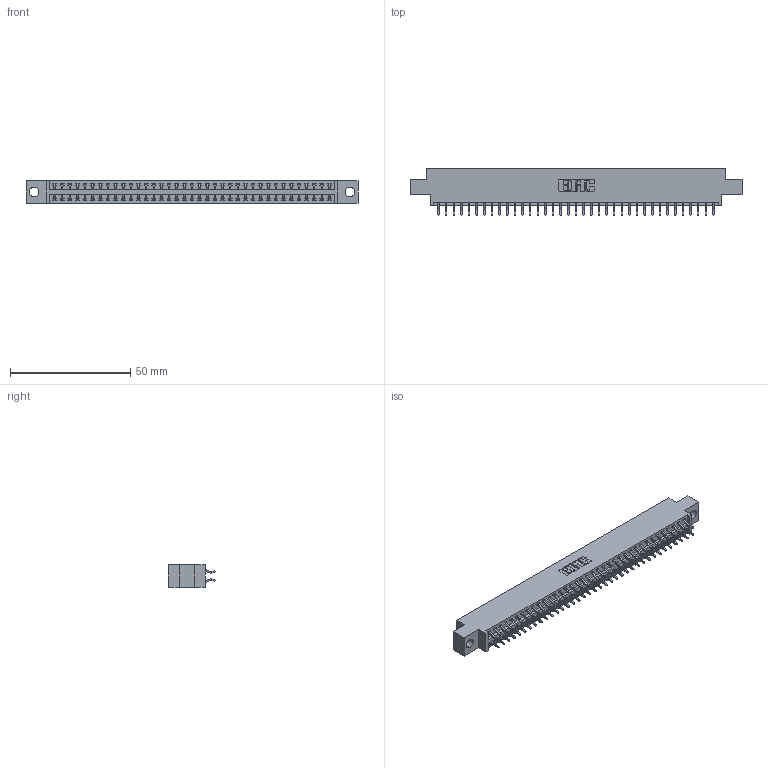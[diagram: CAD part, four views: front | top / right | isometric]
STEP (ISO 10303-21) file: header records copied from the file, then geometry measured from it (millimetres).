
FILE_DESCRIPTION (( 'STEP AP203' ), '1' );
FILE_NAME ('346-074-556-804.STEP', '2022-05-25T03:17:47', ( '' ), ( '' ), 'SwSTEP 2.0', 'SolidWorks 2020', '' );
FILE_SCHEMA (( 'CONFIG_CONTROL_DESIGN' ));
Length unit declared in the file: inch
Products named in the file (3): 345-292-001_556 Tail; 346-074-556-804; 346 Part_0.170 Offset - 0.156 Dia-TH
Assembly tree (75 placements, depth 2):
  346-074-556-804
    346 Part_0.170 Offset - 0.156 Dia-TH
    345-292-001_556 Tail  x74
Bounding box: 138.05 x 19.57 x 9.4 mm (x, y, z)
Volume: 13159.2 mm3; surface area: 17968.3 mm2
Topology: 75 solids, 75 shells, 4432 faces, 13179 edges, 8686 vertices
Faces by surface type: plane 2980, cylinder 1452
Entity records: 25591 total; most frequent: CARTESIAN_POINT 4246, ORIENTED_EDGE 4166, DIRECTION 3779, EDGE_CURVE 2083, VECTOR 1795, LINE 1795, VERTEX_POINT 1386, AXIS2_PLACEMENT_3D 992
